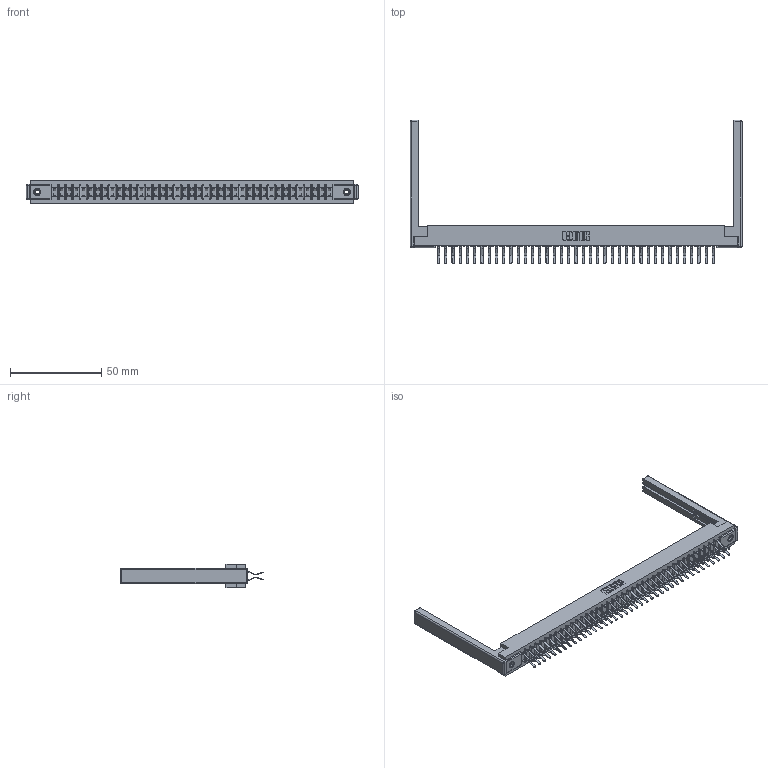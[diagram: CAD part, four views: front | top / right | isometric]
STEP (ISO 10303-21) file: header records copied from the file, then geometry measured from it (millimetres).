
FILE_DESCRIPTION (( 'STEP AP203' ), '1' );
FILE_NAME ('307-078-460-268.STEP', '2020-10-01T07:53:10', ( '' ), ( '' ), 'SwSTEP 2.0', 'SolidWorks 2020', '' );
FILE_SCHEMA (( 'CONFIG_CONTROL_DESIGN' ));
Length unit declared in the file: inch
Products named in the file (5): 307-220-068; 307-078-460-268; 345-250-001_345-250-001-102; 307-290-001_560; 307 Part_.156 Dia Mounting Holes
Assembly tree (83 placements, depth 2):
  307-078-460-268
    307 Part_.156 Dia Mounting Holes
    307-290-001_560  x78
    307-220-068  x2
    345-250-001_345-250-001-102  x2
Bounding box: 181.97 x 78.69 x 12.7 mm (x, y, z)
Volume: 23806.5 mm3; surface area: 28213.5 mm2
Topology: 83 solids, 83 shells, 4212 faces, 11789 edges, 7626 vertices
Faces by surface type: plane 2732, cylinder 1376, sphere 88, cone 12, torus 4
Entity records: 37915 total; most frequent: CARTESIAN_POINT 6180, ORIENTED_EDGE 6116, DIRECTION 6070, EDGE_CURVE 3058, LINE 2342, VECTOR 2342, VERTEX_POINT 1974, AXIS2_PLACEMENT_3D 1864
